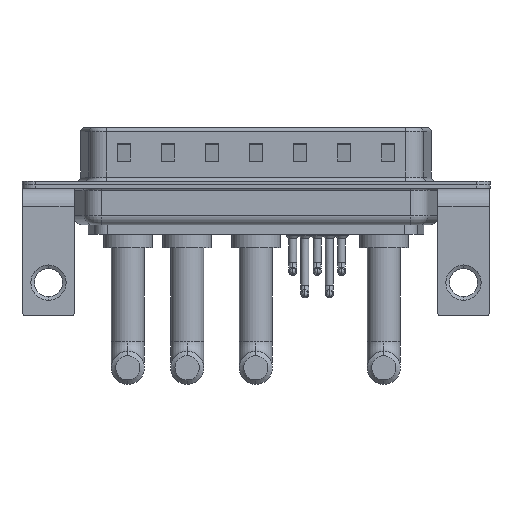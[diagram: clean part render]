
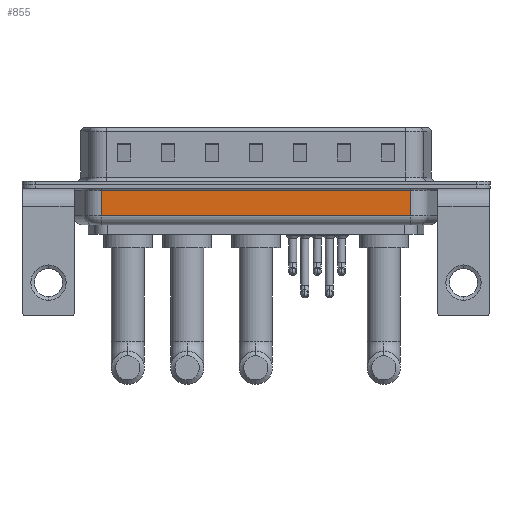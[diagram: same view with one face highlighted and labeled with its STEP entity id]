
A CAD part, front view. The second image highlights one B-rep face of the part: STEP entity #855.
In plain terms, the highlighted planar face has unit normal (0, -1, 0).
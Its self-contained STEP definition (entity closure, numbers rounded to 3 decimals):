
#54 = DIRECTION ( 'NONE',  ( 0., 0., 1. ) ) ;
#60 = CARTESIAN_POINT ( 'NONE',  ( 41.044, -5.35, -0.65 ) ) ;
#129 = DIRECTION ( 'NONE',  ( 0., 1., 0. ) ) ;
#402 = CARTESIAN_POINT ( 'NONE',  ( 6.006, -5.35, -4.5 ) ) ;
#738 = DIRECTION ( 'NONE',  ( 0., 0., 1. ) ) ;
#855 = ADVANCED_FACE ( 'NONE', ( #8836 ), #21370, .F. ) ;
#1443 = EDGE_CURVE ( 'NONE', #1571, #5207, #21815, .T. ) ;
#1571 = VERTEX_POINT ( 'NONE', #60 ) ;
#3026 = ORIENTED_EDGE ( 'NONE', *, *, #20817, .F. ) ;
#3678 = VECTOR ( 'NONE', #5392, 1000. ) ;
#5207 = VERTEX_POINT ( 'NONE', #19587 ) ;
#5392 = DIRECTION ( 'NONE',  ( -1., 0., 0. ) ) ;
#7449 = CARTESIAN_POINT ( 'NONE',  ( 41.044, -5.35, -4.5 ) ) ;
#7647 = DIRECTION ( 'NONE',  ( 0., 0., 1. ) ) ;
#7984 = LINE ( 'NONE', #17110, #11886 ) ;
#8485 = VERTEX_POINT ( 'NONE', #16348 ) ;
#8670 = ORIENTED_EDGE ( 'NONE', *, *, #11102, .T. ) ;
#8836 = FACE_OUTER_BOUND ( 'NONE', #8927, .T. ) ;
#8927 = EDGE_LOOP ( 'NONE', ( #3026, #8670, #20742, #16967 ) ) ;
#9333 = LINE ( 'NONE', #7449, #16889 ) ;
#11033 = CARTESIAN_POINT ( 'NONE',  ( 6.006, -5.35, -0.65 ) ) ;
#11102 = EDGE_CURVE ( 'NONE', #8485, #14502, #7984, .T. ) ;
#11741 = DIRECTION ( 'NONE',  ( 1., 0., 0. ) ) ;
#11886 = VECTOR ( 'NONE', #11741, 1000. ) ;
#12868 = LINE ( 'NONE', #402, #22772 ) ;
#13779 = EDGE_CURVE ( 'NONE', #14502, #1571, #9333, .T. ) ;
#14502 = VERTEX_POINT ( 'NONE', #19358 ) ;
#16348 = CARTESIAN_POINT ( 'NONE',  ( 6.006, -5.35, -3.5 ) ) ;
#16889 = VECTOR ( 'NONE', #738, 1000. ) ;
#16967 = ORIENTED_EDGE ( 'NONE', *, *, #1443, .T. ) ;
#17110 = CARTESIAN_POINT ( 'NONE',  ( 6.006, -5.35, -3.5 ) ) ;
#19358 = CARTESIAN_POINT ( 'NONE',  ( 41.044, -5.35, -3.5 ) ) ;
#19587 = CARTESIAN_POINT ( 'NONE',  ( 6.006, -5.35, -0.65 ) ) ;
#20308 = CARTESIAN_POINT ( 'NONE',  ( 6.006, -5.35, -4.5 ) ) ;
#20742 = ORIENTED_EDGE ( 'NONE', *, *, #13779, .T. ) ;
#20817 = EDGE_CURVE ( 'NONE', #8485, #5207, #12868, .T. ) ;
#21370 = PLANE ( 'NONE',  #22058 ) ;
#21815 = LINE ( 'NONE', #11033, #3678 ) ;
#22058 = AXIS2_PLACEMENT_3D ( 'NONE', #20308, #129, #7647 ) ;
#22772 = VECTOR ( 'NONE', #54, 1000. ) ;
